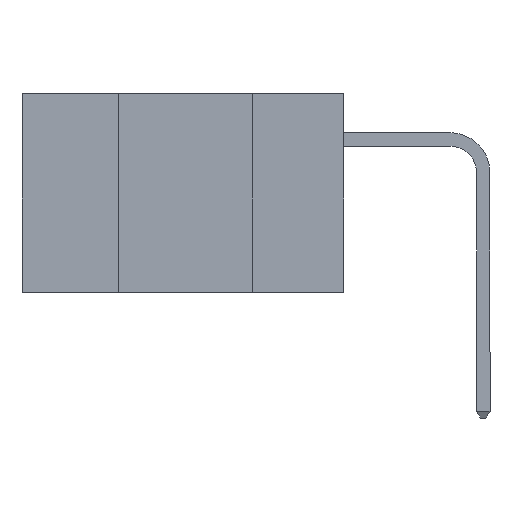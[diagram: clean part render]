
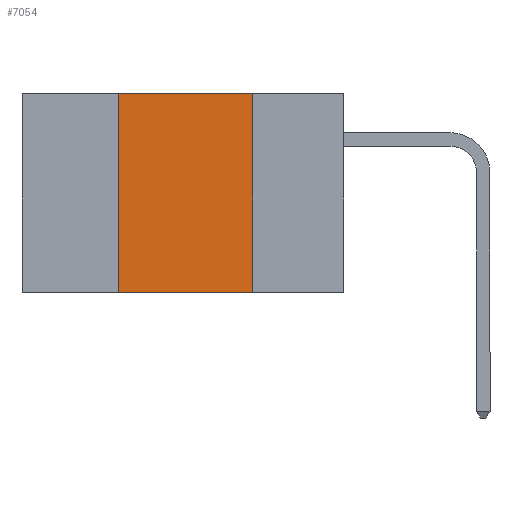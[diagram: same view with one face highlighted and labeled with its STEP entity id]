
A CAD part, left-side view. The second image highlights one B-rep face of the part: STEP entity #7054.
In plain terms, the highlighted planar face has unit normal (-1, 0, 0).
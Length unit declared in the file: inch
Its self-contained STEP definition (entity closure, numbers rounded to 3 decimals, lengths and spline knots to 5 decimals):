
#222 = EDGE_LOOP ( 'NONE', ( #9224, #3107, #6355, #6075 ) ) ;
#378 = CARTESIAN_POINT ( 'NONE',  ( 0., 0.17, -0.37 ) ) ;
#529 = EDGE_CURVE ( 'NONE', #4850, #7359, #7815, .T. ) ;
#630 = AXIS2_PLACEMENT_3D ( 'NONE', #5606, #9211, #6387 ) ;
#1563 = CARTESIAN_POINT ( 'NONE',  ( 0., 0.42, -0.37 ) ) ;
#1692 = FACE_OUTER_BOUND ( 'NONE', #222, .T. ) ;
#2252 = EDGE_CURVE ( 'NONE', #2500, #4850, #5895, .T. ) ;
#2296 = VECTOR ( 'NONE', #7328, 39.37008 ) ;
#2445 = VECTOR ( 'NONE', #2850, 39.37008 ) ;
#2450 = DIRECTION ( 'NONE',  ( 0., -1., 0. ) ) ;
#2500 = VERTEX_POINT ( 'NONE', #9100 ) ;
#2850 = DIRECTION ( 'NONE',  ( 0., -1., 0. ) ) ;
#3107 = ORIENTED_EDGE ( 'NONE', *, *, #2252, .F. ) ;
#3188 = LINE ( 'NONE', #6216, #8932 ) ;
#3469 = EDGE_CURVE ( 'NONE', #4064, #2500, #8138, .T. ) ;
#3705 = EDGE_CURVE ( 'NONE', #4064, #7359, #3188, .T. ) ;
#4064 = VERTEX_POINT ( 'NONE', #1563 ) ;
#4812 = PLANE ( 'NONE',  #630 ) ;
#4850 = VERTEX_POINT ( 'NONE', #5816 ) ;
#5606 = CARTESIAN_POINT ( 'NONE',  ( 0., 0.6, 0. ) ) ;
#5731 = VECTOR ( 'NONE', #6220, 39.37008 ) ;
#5816 = CARTESIAN_POINT ( 'NONE',  ( 0., 0.17, 0. ) ) ;
#5895 = LINE ( 'NONE', #8816, #2445 ) ;
#5988 = CARTESIAN_POINT ( 'NONE',  ( 0., 0.42, -0.37 ) ) ;
#6075 = ORIENTED_EDGE ( 'NONE', *, *, #3705, .T. ) ;
#6216 = CARTESIAN_POINT ( 'NONE',  ( 0., 0.6, -0.37 ) ) ;
#6220 = DIRECTION ( 'NONE',  ( 0., 0., -1. ) ) ;
#6355 = ORIENTED_EDGE ( 'NONE', *, *, #3469, .F. ) ;
#6387 = DIRECTION ( 'NONE',  ( 0., 0., -1. ) ) ;
#7054 = ADVANCED_FACE ( 'NONE', ( #1692 ), #4812, .F. ) ;
#7328 = DIRECTION ( 'NONE',  ( 0., 0., 1. ) ) ;
#7359 = VERTEX_POINT ( 'NONE', #7433 ) ;
#7433 = CARTESIAN_POINT ( 'NONE',  ( 0., 0.17, -0.37 ) ) ;
#7815 = LINE ( 'NONE', #378, #5731 ) ;
#8138 = LINE ( 'NONE', #5988, #2296 ) ;
#8816 = CARTESIAN_POINT ( 'NONE',  ( 0., 0.6, 0. ) ) ;
#8932 = VECTOR ( 'NONE', #2450, 39.37008 ) ;
#9100 = CARTESIAN_POINT ( 'NONE',  ( 0., 0.42, 0. ) ) ;
#9211 = DIRECTION ( 'NONE',  ( 1., 0., 0. ) ) ;
#9224 = ORIENTED_EDGE ( 'NONE', *, *, #529, .F. ) ;
